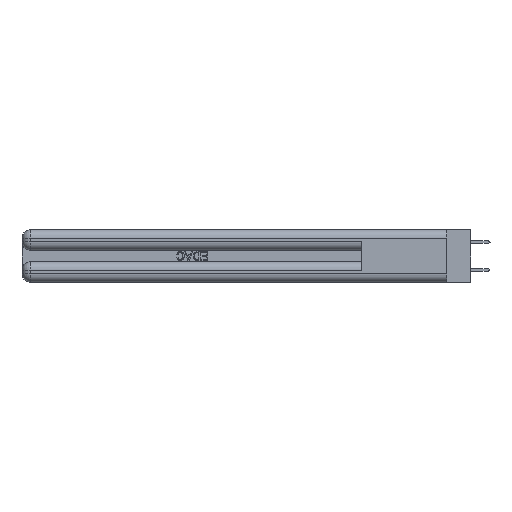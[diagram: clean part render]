
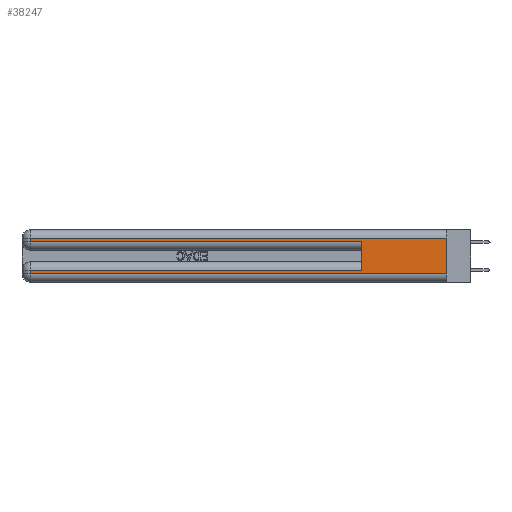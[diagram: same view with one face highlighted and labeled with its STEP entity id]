
A CAD part, left-side view. The second image highlights one B-rep face of the part: STEP entity #38247.
In plain terms, the highlighted planar face has unit normal (-1, 0, 0).
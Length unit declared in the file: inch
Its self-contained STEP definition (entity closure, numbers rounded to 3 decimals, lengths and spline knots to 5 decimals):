
#171 = CARTESIAN_POINT ( 'NONE',  ( 0., 2.94, 0.06 ) ) ;
#1348 = DIRECTION ( 'NONE',  ( 1., 0., 0. ) ) ;
#2504 = VECTOR ( 'NONE', #27434, 39.37008 ) ;
#3203 = LINE ( 'NONE', #16909, #8921 ) ;
#3447 = VERTEX_POINT ( 'NONE', #14290 ) ;
#4435 = CARTESIAN_POINT ( 'NONE',  ( 0., 0., 0.37 ) ) ;
#4554 = ORIENTED_EDGE ( 'NONE', *, *, #41841, .T. ) ;
#4569 = EDGE_CURVE ( 'NONE', #17951, #30253, #15263, .T. ) ;
#4915 = PLANE ( 'NONE',  #37280 ) ;
#5020 = VERTEX_POINT ( 'NONE', #48246 ) ;
#5731 = LINE ( 'NONE', #33121, #44650 ) ;
#5896 = ORIENTED_EDGE ( 'NONE', *, *, #43074, .F. ) ;
#6972 = CARTESIAN_POINT ( 'NONE',  ( 0., 2.94, 0.31 ) ) ;
#7385 = CARTESIAN_POINT ( 'NONE',  ( 0., 0., 0.06 ) ) ;
#8176 = VERTEX_POINT ( 'NONE', #27568 ) ;
#8845 = CARTESIAN_POINT ( 'NONE',  ( 0., 2.94, 0.085 ) ) ;
#8921 = VECTOR ( 'NONE', #20750, 39.37008 ) ;
#10742 = CARTESIAN_POINT ( 'NONE',  ( 0., 0.6, 0.145 ) ) ;
#11241 = CARTESIAN_POINT ( 'NONE',  ( 0., 0., 0.31 ) ) ;
#11508 = LINE ( 'NONE', #10742, #29109 ) ;
#11539 = EDGE_LOOP ( 'NONE', ( #5896, #13326, #4554, #15185, #41990, #24988, #18184, #49622 ) ) ;
#12823 = CARTESIAN_POINT ( 'NONE',  ( 0., 0.6, 0.085 ) ) ;
#13326 = ORIENTED_EDGE ( 'NONE', *, *, #21175, .T. ) ;
#14225 = VECTOR ( 'NONE', #46374, 39.37008 ) ;
#14290 = CARTESIAN_POINT ( 'NONE',  ( 0., 2.94, 0.285 ) ) ;
#14359 = EDGE_CURVE ( 'NONE', #3447, #8176, #39092, .T. ) ;
#14796 = EDGE_CURVE ( 'NONE', #27370, #48522, #3203, .T. ) ;
#15158 = LINE ( 'NONE', #4435, #27803 ) ;
#15185 = ORIENTED_EDGE ( 'NONE', *, *, #14359, .T. ) ;
#15254 = CARTESIAN_POINT ( 'NONE',  ( 0., 2.94, 0.37 ) ) ;
#15263 = LINE ( 'NONE', #7385, #2504 ) ;
#15493 = LINE ( 'NONE', #15254, #14225 ) ;
#16909 = CARTESIAN_POINT ( 'NONE',  ( 0., 0., 0.085 ) ) ;
#17951 = VERTEX_POINT ( 'NONE', #171 ) ;
#18184 = ORIENTED_EDGE ( 'NONE', *, *, #46893, .T. ) ;
#20375 = DIRECTION ( 'NONE',  ( 0., 0., -1. ) ) ;
#20750 = DIRECTION ( 'NONE',  ( 0., 1., 0. ) ) ;
#21175 = EDGE_CURVE ( 'NONE', #5020, #43427, #42378, .T. ) ;
#22926 = VECTOR ( 'NONE', #45657, 39.37008 ) ;
#24513 = CARTESIAN_POINT ( 'NONE',  ( 0., 0., 0.37 ) ) ;
#24988 = ORIENTED_EDGE ( 'NONE', *, *, #14796, .T. ) ;
#26002 = DIRECTION ( 'NONE',  ( 0., 0., 1. ) ) ;
#26349 = CARTESIAN_POINT ( 'NONE',  ( 0., 0., 0.06 ) ) ;
#26528 = CARTESIAN_POINT ( 'NONE',  ( 0., 0., 0.285 ) ) ;
#27370 = VERTEX_POINT ( 'NONE', #12823 ) ;
#27434 = DIRECTION ( 'NONE',  ( 0., -1., 0. ) ) ;
#27568 = CARTESIAN_POINT ( 'NONE',  ( 0., 0.6, 0.285 ) ) ;
#27803 = VECTOR ( 'NONE', #46003, 39.37008 ) ;
#28073 = DIRECTION ( 'NONE',  ( 0., 0., -1. ) ) ;
#29109 = VECTOR ( 'NONE', #26002, 39.37008 ) ;
#30253 = VERTEX_POINT ( 'NONE', #26349 ) ;
#30777 = DIRECTION ( 'NONE',  ( 0., -1., 0. ) ) ;
#33121 = CARTESIAN_POINT ( 'NONE',  ( 0., 2.94, 0.37 ) ) ;
#35369 = FACE_OUTER_BOUND ( 'NONE', #11539, .T. ) ;
#35954 = EDGE_CURVE ( 'NONE', #27370, #8176, #11508, .T. ) ;
#37280 = AXIS2_PLACEMENT_3D ( 'NONE', #24513, #1348, #28073 ) ;
#38247 = ADVANCED_FACE ( 'NONE', ( #35369 ), #4915, .F. ) ;
#39092 = LINE ( 'NONE', #26528, #39577 ) ;
#39577 = VECTOR ( 'NONE', #30777, 39.37008 ) ;
#41841 = EDGE_CURVE ( 'NONE', #43427, #3447, #5731, .T. ) ;
#41990 = ORIENTED_EDGE ( 'NONE', *, *, #35954, .F. ) ;
#42378 = LINE ( 'NONE', #11241, #22926 ) ;
#43074 = EDGE_CURVE ( 'NONE', #5020, #30253, #15158, .T. ) ;
#43427 = VERTEX_POINT ( 'NONE', #6972 ) ;
#44650 = VECTOR ( 'NONE', #20375, 39.37008 ) ;
#45657 = DIRECTION ( 'NONE',  ( 0., 1., 0. ) ) ;
#46003 = DIRECTION ( 'NONE',  ( 0., 0., -1. ) ) ;
#46374 = DIRECTION ( 'NONE',  ( 0., 0., -1. ) ) ;
#46893 = EDGE_CURVE ( 'NONE', #48522, #17951, #15493, .T. ) ;
#48246 = CARTESIAN_POINT ( 'NONE',  ( 0., 0., 0.31 ) ) ;
#48522 = VERTEX_POINT ( 'NONE', #8845 ) ;
#49622 = ORIENTED_EDGE ( 'NONE', *, *, #4569, .T. ) ;
